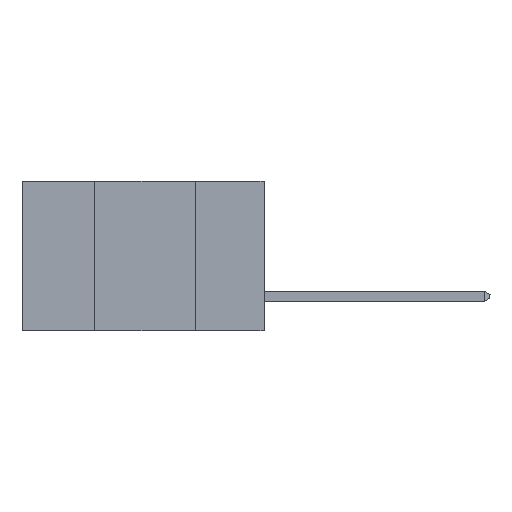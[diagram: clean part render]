
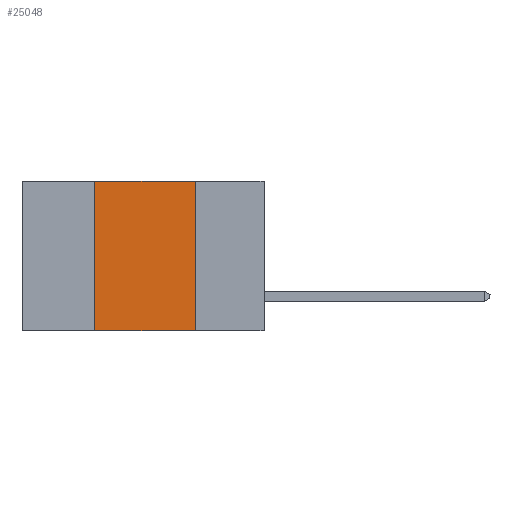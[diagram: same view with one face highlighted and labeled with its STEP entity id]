
A CAD part, left-side view. The second image highlights one B-rep face of the part: STEP entity #25048.
In plain terms, the highlighted planar face has unit normal (-1, 0, 0).
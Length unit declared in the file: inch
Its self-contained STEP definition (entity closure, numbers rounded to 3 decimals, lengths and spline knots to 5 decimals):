
#25 = LINE ( 'NONE', #19953, #11294 ) ;
#667 = DIRECTION ( 'NONE',  ( 0., 0., -1. ) ) ;
#1102 = VERTEX_POINT ( 'NONE', #18547 ) ;
#1242 = VECTOR ( 'NONE', #1316, 39.37008 ) ;
#1316 = DIRECTION ( 'NONE',  ( 0., 0., -1. ) ) ;
#6143 = VECTOR ( 'NONE', #13943, 39.37008 ) ;
#6753 = CARTESIAN_POINT ( 'NONE',  ( 0., 0.42, -0.37 ) ) ;
#9256 = CARTESIAN_POINT ( 'NONE',  ( 0., 0.6, -0.37 ) ) ;
#10393 = ORIENTED_EDGE ( 'NONE', *, *, #22133, .F. ) ;
#11146 = EDGE_LOOP ( 'NONE', ( #19942, #10393, #13321, #22957 ) ) ;
#11294 = VECTOR ( 'NONE', #19823, 39.37008 ) ;
#12270 = EDGE_CURVE ( 'NONE', #23278, #21777, #16613, .T. ) ;
#12367 = EDGE_CURVE ( 'NONE', #1102, #23798, #23082, .T. ) ;
#12860 = CARTESIAN_POINT ( 'NONE',  ( 0., 0.17, -0.37 ) ) ;
#13321 = ORIENTED_EDGE ( 'NONE', *, *, #12270, .F. ) ;
#13750 = CARTESIAN_POINT ( 'NONE',  ( 0., 0.42, -0.37 ) ) ;
#13943 = DIRECTION ( 'NONE',  ( 0., 0., 1. ) ) ;
#15102 = LINE ( 'NONE', #9256, #15822 ) ;
#15822 = VECTOR ( 'NONE', #21181, 39.37008 ) ;
#16332 = CARTESIAN_POINT ( 'NONE',  ( 0., 0.6, 0. ) ) ;
#16613 = LINE ( 'NONE', #6753, #6143 ) ;
#17108 = CARTESIAN_POINT ( 'NONE',  ( 0., 0.42, 0. ) ) ;
#18280 = DIRECTION ( 'NONE',  ( 1., 0., 0. ) ) ;
#18547 = CARTESIAN_POINT ( 'NONE',  ( 0., 0.17, 0. ) ) ;
#19823 = DIRECTION ( 'NONE',  ( 0., -1., 0. ) ) ;
#19929 = CARTESIAN_POINT ( 'NONE',  ( 0., 0.17, -0.37 ) ) ;
#19942 = ORIENTED_EDGE ( 'NONE', *, *, #12367, .F. ) ;
#19953 = CARTESIAN_POINT ( 'NONE',  ( 0., 0.6, 0. ) ) ;
#20213 = PLANE ( 'NONE',  #21696 ) ;
#20463 = FACE_OUTER_BOUND ( 'NONE', #11146, .T. ) ;
#20911 = EDGE_CURVE ( 'NONE', #23278, #23798, #15102, .T. ) ;
#21181 = DIRECTION ( 'NONE',  ( 0., -1., 0. ) ) ;
#21696 = AXIS2_PLACEMENT_3D ( 'NONE', #16332, #18280, #667 ) ;
#21777 = VERTEX_POINT ( 'NONE', #17108 ) ;
#22133 = EDGE_CURVE ( 'NONE', #21777, #1102, #25, .T. ) ;
#22957 = ORIENTED_EDGE ( 'NONE', *, *, #20911, .T. ) ;
#23082 = LINE ( 'NONE', #12860, #1242 ) ;
#23278 = VERTEX_POINT ( 'NONE', #13750 ) ;
#23798 = VERTEX_POINT ( 'NONE', #19929 ) ;
#25048 = ADVANCED_FACE ( 'NONE', ( #20463 ), #20213, .F. ) ;
